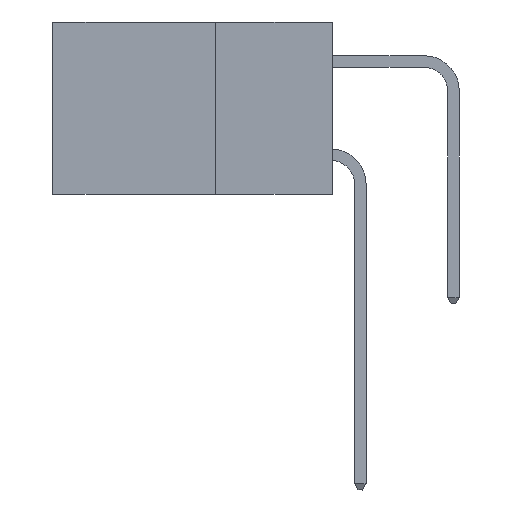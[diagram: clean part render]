
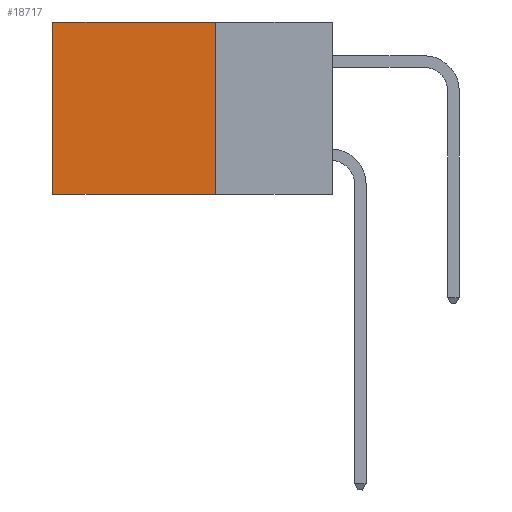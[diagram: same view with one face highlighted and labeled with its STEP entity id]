
A CAD part, left-side view. The second image highlights one B-rep face of the part: STEP entity #18717.
In plain terms, the highlighted planar face has unit normal (-1, 0, 0).
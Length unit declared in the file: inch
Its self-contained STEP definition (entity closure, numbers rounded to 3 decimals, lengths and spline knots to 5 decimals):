
#2637 = VECTOR ( 'NONE', #6918, 39.37008 ) ;
#2824 = DIRECTION ( 'NONE',  ( 0., 1., 0. ) ) ;
#3098 = CARTESIAN_POINT ( 'NONE',  ( 0.298, 0.6, 0. ) ) ;
#5082 = EDGE_CURVE ( 'NONE', #14893, #17437, #8106, .T. ) ;
#5227 = LINE ( 'NONE', #9984, #11824 ) ;
#5259 = CARTESIAN_POINT ( 'NONE',  ( 0.298, 0.25, 0. ) ) ;
#6480 = VECTOR ( 'NONE', #10793, 39.37008 ) ;
#6918 = DIRECTION ( 'NONE',  ( 0., 1., 0. ) ) ;
#6986 = CARTESIAN_POINT ( 'NONE',  ( 0.298, 0.25, 0. ) ) ;
#7927 = AXIS2_PLACEMENT_3D ( 'NONE', #5259, #15263, #15394 ) ;
#8106 = LINE ( 'NONE', #6986, #2637 ) ;
#8238 = ORIENTED_EDGE ( 'NONE', *, *, #5082, .T. ) ;
#8760 = FACE_OUTER_BOUND ( 'NONE', #10547, .T. ) ;
#8792 = ORIENTED_EDGE ( 'NONE', *, *, #17589, .F. ) ;
#8834 = CARTESIAN_POINT ( 'NONE',  ( 0.298, 0.6, -0.37 ) ) ;
#8993 = LINE ( 'NONE', #16322, #6480 ) ;
#9122 = ORIENTED_EDGE ( 'NONE', *, *, #9997, .F. ) ;
#9179 = VERTEX_POINT ( 'NONE', #13581 ) ;
#9984 = CARTESIAN_POINT ( 'NONE',  ( 0.298, 0.6, 0. ) ) ;
#9997 = EDGE_CURVE ( 'NONE', #9179, #14136, #15160, .T. ) ;
#10052 = CARTESIAN_POINT ( 'NONE',  ( 0.298, 0.25, 0. ) ) ;
#10547 = EDGE_LOOP ( 'NONE', ( #17460, #9122, #8792, #8238 ) ) ;
#10793 = DIRECTION ( 'NONE',  ( 0., 0., -1. ) ) ;
#11466 = CARTESIAN_POINT ( 'NONE',  ( 0.298, 0.25, -0.37 ) ) ;
#11824 = VECTOR ( 'NONE', #15914, 39.37008 ) ;
#12253 = EDGE_CURVE ( 'NONE', #17437, #14136, #5227, .T. ) ;
#13152 = VECTOR ( 'NONE', #2824, 39.37008 ) ;
#13581 = CARTESIAN_POINT ( 'NONE',  ( 0.298, 0.25, -0.37 ) ) ;
#14136 = VERTEX_POINT ( 'NONE', #8834 ) ;
#14893 = VERTEX_POINT ( 'NONE', #10052 ) ;
#15160 = LINE ( 'NONE', #11466, #13152 ) ;
#15263 = DIRECTION ( 'NONE',  ( 1., 0., 0. ) ) ;
#15394 = DIRECTION ( 'NONE',  ( 0., 0., -1. ) ) ;
#15914 = DIRECTION ( 'NONE',  ( 0., 0., -1. ) ) ;
#16322 = CARTESIAN_POINT ( 'NONE',  ( 0.298, 0.25, 0. ) ) ;
#16330 = PLANE ( 'NONE',  #7927 ) ;
#17437 = VERTEX_POINT ( 'NONE', #3098 ) ;
#17460 = ORIENTED_EDGE ( 'NONE', *, *, #12253, .T. ) ;
#17589 = EDGE_CURVE ( 'NONE', #14893, #9179, #8993, .T. ) ;
#18717 = ADVANCED_FACE ( 'NONE', ( #8760 ), #16330, .F. ) ;
